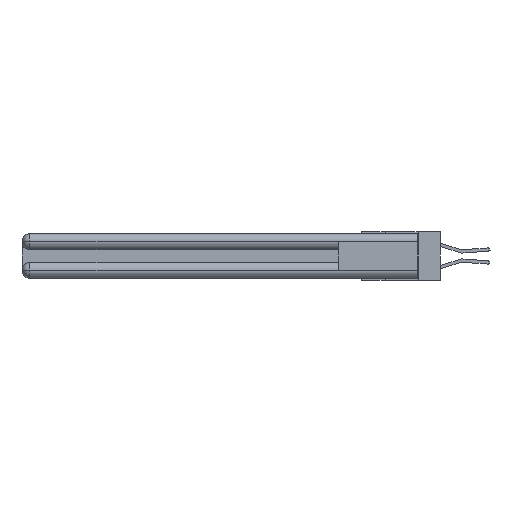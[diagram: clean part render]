
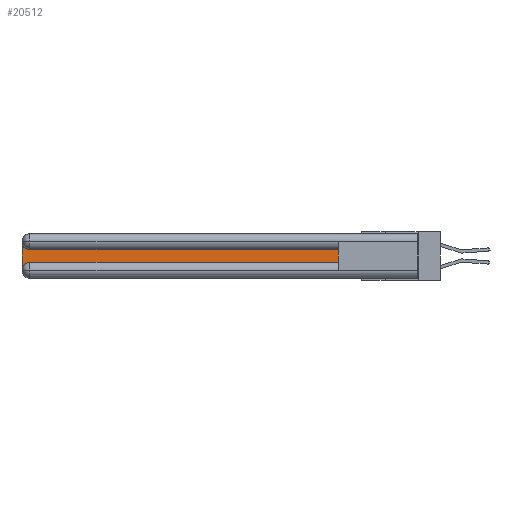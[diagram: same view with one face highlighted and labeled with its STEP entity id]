
A CAD part, left-side view. The second image highlights one B-rep face of the part: STEP entity #20512.
In plain terms, the highlighted planar face has unit normal (-1, 0, 0).
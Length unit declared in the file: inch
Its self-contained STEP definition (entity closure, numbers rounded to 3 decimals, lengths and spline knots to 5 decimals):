
#780 = ORIENTED_EDGE ( 'NONE', *, *, #18402, .T. ) ;
#1669 = VERTEX_POINT ( 'NONE', #9098 ) ;
#1870 = VECTOR ( 'NONE', #3268, 39.37008 ) ;
#2511 = CARTESIAN_POINT ( 'NONE',  ( 0.075, 0.6, -0.1225 ) ) ;
#2938 = DIRECTION ( 'NONE',  ( 0., 0., -1. ) ) ;
#3268 = DIRECTION ( 'NONE',  ( 0., 0., 1. ) ) ;
#3714 = AXIS2_PLACEMENT_3D ( 'NONE', #24137, #21460, #27021 ) ;
#3891 = ORIENTED_EDGE ( 'NONE', *, *, #24138, .T. ) ;
#3960 = CIRCLE ( 'NONE', #23097, 0.06 ) ;
#4271 = FACE_OUTER_BOUND ( 'NONE', #11133, .T. ) ;
#4720 = ORIENTED_EDGE ( 'NONE', *, *, #11819, .T. ) ;
#6842 = LINE ( 'NONE', #22292, #32433 ) ;
#7343 = EDGE_CURVE ( 'NONE', #22748, #1669, #11867, .T. ) ;
#7868 = CARTESIAN_POINT ( 'NONE',  ( 0.075, 2.94, -0.2775 ) ) ;
#8560 = CARTESIAN_POINT ( 'NONE',  ( 0.075, 0.6, -0.2175 ) ) ;
#9098 = CARTESIAN_POINT ( 'NONE',  ( 0.075, 2.94, -0.1225 ) ) ;
#11133 = EDGE_LOOP ( 'NONE', ( #33105, #780, #23834, #4720, #30161, #3891 ) ) ;
#11306 = DIRECTION ( 'NONE',  ( 0., 1., 0. ) ) ;
#11819 = EDGE_CURVE ( 'NONE', #20348, #24318, #18651, .T. ) ;
#11867 = LINE ( 'NONE', #27120, #31670 ) ;
#11901 = VERTEX_POINT ( 'NONE', #27465 ) ;
#12716 = DIRECTION ( 'NONE',  ( 1., 0., 0. ) ) ;
#15817 = DIRECTION ( 'NONE',  ( 0., 0., -1. ) ) ;
#16048 = DIRECTION ( 'NONE',  ( 1., 0., 0. ) ) ;
#17598 = VECTOR ( 'NONE', #2938, 39.37008 ) ;
#18148 = DIRECTION ( 'NONE',  ( 0., 0., -1. ) ) ;
#18402 = EDGE_CURVE ( 'NONE', #1669, #24598, #3960, .T. ) ;
#18405 = CARTESIAN_POINT ( 'NONE',  ( 0.075, 3., -0.2175 ) ) ;
#18651 = CIRCLE ( 'NONE', #31879, 0.06 ) ;
#20348 = VERTEX_POINT ( 'NONE', #33516 ) ;
#20512 = ADVANCED_FACE ( 'NONE', ( #4271 ), #32448, .F. ) ;
#21460 = DIRECTION ( 'NONE',  ( 1., 0., 0. ) ) ;
#22292 = CARTESIAN_POINT ( 'NONE',  ( 0.075, 0.6, -0.2175 ) ) ;
#22746 = DIRECTION ( 'NONE',  ( 0., -1., 0. ) ) ;
#22748 = VERTEX_POINT ( 'NONE', #2511 ) ;
#23097 = AXIS2_PLACEMENT_3D ( 'NONE', #26336, #16048, #15817 ) ;
#23655 = CARTESIAN_POINT ( 'NONE',  ( 0.075, 3., -0.0625 ) ) ;
#23834 = ORIENTED_EDGE ( 'NONE', *, *, #31378, .T. ) ;
#24137 = CARTESIAN_POINT ( 'NONE',  ( 0.075, 3., -0.1225 ) ) ;
#24138 = EDGE_CURVE ( 'NONE', #11901, #22748, #30333, .T. ) ;
#24175 = LINE ( 'NONE', #18405, #17598 ) ;
#24318 = VERTEX_POINT ( 'NONE', #27486 ) ;
#24598 = VERTEX_POINT ( 'NONE', #23655 ) ;
#26336 = CARTESIAN_POINT ( 'NONE',  ( 0.075, 2.94, -0.0625 ) ) ;
#27021 = DIRECTION ( 'NONE',  ( 0., 0., -1. ) ) ;
#27120 = CARTESIAN_POINT ( 'NONE',  ( 0.075, 0.6, -0.1225 ) ) ;
#27465 = CARTESIAN_POINT ( 'NONE',  ( 0.075, 0.6, -0.2175 ) ) ;
#27486 = CARTESIAN_POINT ( 'NONE',  ( 0.075, 2.94, -0.2175 ) ) ;
#30161 = ORIENTED_EDGE ( 'NONE', *, *, #31718, .T. ) ;
#30333 = LINE ( 'NONE', #8560, #1870 ) ;
#31378 = EDGE_CURVE ( 'NONE', #24598, #20348, #24175, .T. ) ;
#31670 = VECTOR ( 'NONE', #11306, 39.37008 ) ;
#31718 = EDGE_CURVE ( 'NONE', #24318, #11901, #6842, .T. ) ;
#31879 = AXIS2_PLACEMENT_3D ( 'NONE', #7868, #12716, #18148 ) ;
#32433 = VECTOR ( 'NONE', #22746, 39.37008 ) ;
#32448 = PLANE ( 'NONE',  #3714 ) ;
#33105 = ORIENTED_EDGE ( 'NONE', *, *, #7343, .T. ) ;
#33516 = CARTESIAN_POINT ( 'NONE',  ( 0.075, 3., -0.2775 ) ) ;
